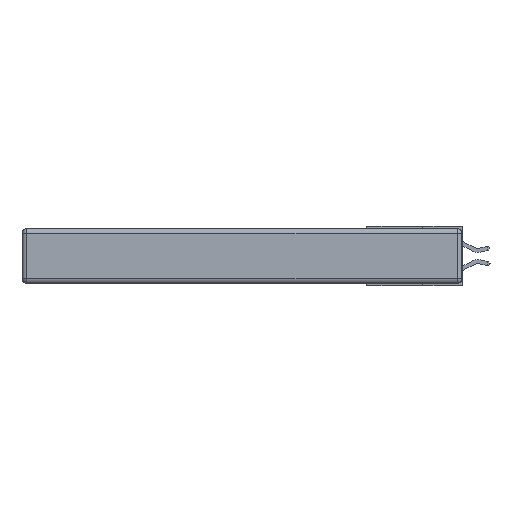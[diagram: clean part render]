
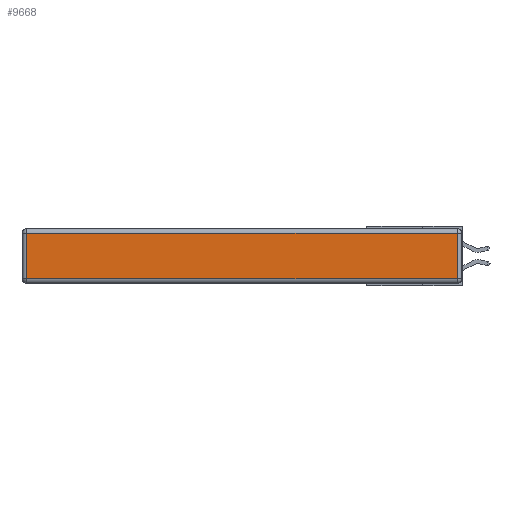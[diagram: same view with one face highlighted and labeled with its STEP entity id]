
A CAD part, left-side view. The second image highlights one B-rep face of the part: STEP entity #9668.
In plain terms, the highlighted planar face has unit normal (-1, 0, 0).
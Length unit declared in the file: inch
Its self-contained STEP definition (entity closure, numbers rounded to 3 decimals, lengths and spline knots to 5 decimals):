
#1485 = DIRECTION ( 'NONE',  ( 0., 0., 1. ) ) ;
#1523 = PLANE ( 'NONE',  #10327 ) ;
#1793 = DIRECTION ( 'NONE',  ( 0., 0., -1. ) ) ;
#1904 = CARTESIAN_POINT ( 'NONE',  ( 0., 0., -0.313 ) ) ;
#3346 = CARTESIAN_POINT ( 'NONE',  ( 0., 2.72, -0.313 ) ) ;
#5969 = CARTESIAN_POINT ( 'NONE',  ( 0., 2.72, -0.03 ) ) ;
#6472 = EDGE_LOOP ( 'NONE', ( #28418, #16517, #21145, #21598 ) ) ;
#7848 = CARTESIAN_POINT ( 'NONE',  ( 0., 0., -0.343 ) ) ;
#8616 = DIRECTION ( 'NONE',  ( 0., -1., 0. ) ) ;
#8680 = VECTOR ( 'NONE', #8616, 39.37008 ) ;
#9668 = ADVANCED_FACE ( 'NONE', ( #18781 ), #1523, .T. ) ;
#10327 = AXIS2_PLACEMENT_3D ( 'NONE', #7848, #18757, #16943 ) ;
#10984 = VECTOR ( 'NONE', #1485, 39.37008 ) ;
#11324 = VERTEX_POINT ( 'NONE', #17501 ) ;
#12741 = VERTEX_POINT ( 'NONE', #17669 ) ;
#15557 = DIRECTION ( 'NONE',  ( 0., 1., 0. ) ) ;
#15937 = CARTESIAN_POINT ( 'NONE',  ( 0., 2.75, -0.03 ) ) ;
#16078 = LINE ( 'NONE', #19030, #23244 ) ;
#16463 = EDGE_CURVE ( 'NONE', #11324, #12741, #21331, .T. ) ;
#16517 = ORIENTED_EDGE ( 'NONE', *, *, #16463, .T. ) ;
#16943 = DIRECTION ( 'NONE',  ( 0., 0., 1. ) ) ;
#17246 = VERTEX_POINT ( 'NONE', #3346 ) ;
#17501 = CARTESIAN_POINT ( 'NONE',  ( 0., 0.03, -0.313 ) ) ;
#17669 = CARTESIAN_POINT ( 'NONE',  ( 0., 0.03, -0.03 ) ) ;
#18757 = DIRECTION ( 'NONE',  ( -1., 0., 0. ) ) ;
#18781 = FACE_OUTER_BOUND ( 'NONE', #6472, .T. ) ;
#18819 = VERTEX_POINT ( 'NONE', #5969 ) ;
#19030 = CARTESIAN_POINT ( 'NONE',  ( 0., 2.72, -0.343 ) ) ;
#19226 = VECTOR ( 'NONE', #15557, 39.37008 ) ;
#19303 = EDGE_CURVE ( 'NONE', #17246, #11324, #26540, .T. ) ;
#20396 = CARTESIAN_POINT ( 'NONE',  ( 0., 0.03, -0.343 ) ) ;
#21145 = ORIENTED_EDGE ( 'NONE', *, *, #21660, .T. ) ;
#21331 = LINE ( 'NONE', #20396, #10984 ) ;
#21598 = ORIENTED_EDGE ( 'NONE', *, *, #24008, .T. ) ;
#21660 = EDGE_CURVE ( 'NONE', #12741, #18819, #25031, .T. ) ;
#23244 = VECTOR ( 'NONE', #1793, 39.37008 ) ;
#24008 = EDGE_CURVE ( 'NONE', #18819, #17246, #16078, .T. ) ;
#25031 = LINE ( 'NONE', #15937, #19226 ) ;
#26540 = LINE ( 'NONE', #1904, #8680 ) ;
#28418 = ORIENTED_EDGE ( 'NONE', *, *, #19303, .T. ) ;
